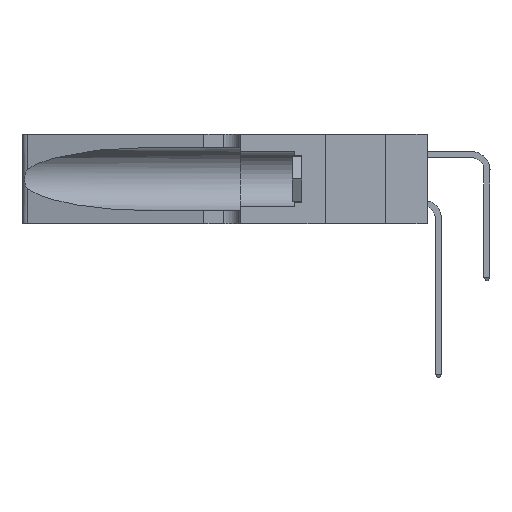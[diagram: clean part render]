
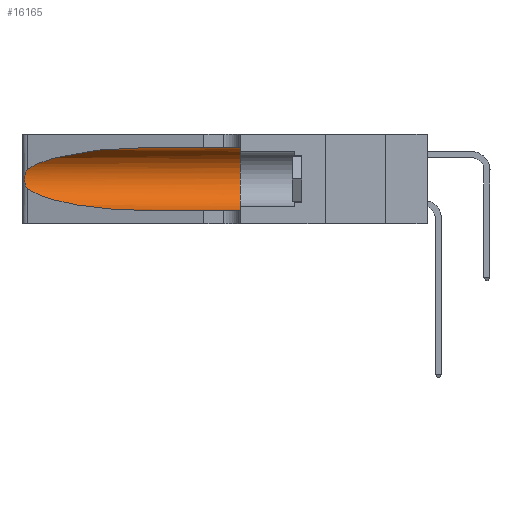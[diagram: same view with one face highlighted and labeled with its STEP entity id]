
A CAD part, left-side view. The second image highlights one B-rep face of the part: STEP entity #16165.
In plain terms, the highlighted cylindrical face has radius 3.308 mm (diameter 6.617 mm), a partial arc.
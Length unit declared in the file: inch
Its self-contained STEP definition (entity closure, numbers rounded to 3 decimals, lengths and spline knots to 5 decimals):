
#218 = VECTOR ( 'NONE', #19047, 39.37008 ) ;
#961 = LINE ( 'NONE', #16708, #218 ) ;
#1011 = B_SPLINE_CURVE_WITH_KNOTS ( 'NONE', 3,
 ( #8698, #10988, #27012, #13292, #29279, #15613, #1794, #17951, #4158, #20252, #6467, #22517, #8791, #24831 ),
 .UNSPECIFIED., .F., .F.,
 ( 4, 2, 2, 2, 2, 2, 4 ),
 ( 0., 0.00027, 0.00053, 0.00107, 0.0016, 0.00187, 0.00214 ),
 .UNSPECIFIED. ) ;
#1794 = CARTESIAN_POINT ( 'NONE',  ( 0.26075, 1.23896, 0.19203 ) ) ;
#2003 = EDGE_LOOP ( 'NONE', ( #27450, #5234, #14921, #28518, #14571, #28187 ) ) ;
#2371 = CARTESIAN_POINT ( 'NONE',  ( 0.2373, 1.15595, 0.08982 ) ) ;
#3690 = FACE_OUTER_BOUND ( 'NONE', #2003, .T. ) ;
#4009 = DIRECTION ( 'NONE',  ( 0., -1., 0. ) ) ;
#4158 = CARTESIAN_POINT ( 'NONE',  ( 0.26017, 1.23833, 0.17102 ) ) ;
#4288 = VECTOR ( 'NONE', #4009, 39.37008 ) ;
#4732 = CARTESIAN_POINT ( 'NONE',  ( 0.25487, 1.22718, 0.14631 ) ) ;
#4951 = AXIS2_PLACEMENT_3D ( 'NONE', #19321, #5542, #21601 ) ;
#5097 = VERTEX_POINT ( 'NONE', #6331 ) ;
#5208 = AXIS2_PLACEMENT_3D ( 'NONE', #8575, #22300, #10869 ) ;
#5234 = ORIENTED_EDGE ( 'NONE', *, *, #7033, .T. ) ;
#5542 = DIRECTION ( 'NONE',  ( 0., 1., 0. ) ) ;
#6032 = CARTESIAN_POINT ( 'NONE',  ( 0.1305, 0.35, 0.31525 ) ) ;
#6320 = VERTEX_POINT ( 'NONE', #28632 ) ;
#6331 = CARTESIAN_POINT ( 'NONE',  ( 0.25487, 1.22718, 0.14631 ) ) ;
#6467 = CARTESIAN_POINT ( 'NONE',  ( 0.25789, 1.23486, 0.15765 ) ) ;
#7033 = EDGE_CURVE ( 'NONE', #21579, #5097, #1011, .T. ) ;
#7039 = CARTESIAN_POINT ( 'NONE',  ( 0.18966, 0.96281, 0.05475 ) ) ;
#7340 =( BOUNDED_CURVE ( )  B_SPLINE_CURVE ( 3, ( #4732, #2371, #7039, #23074 ),
 .UNSPECIFIED., .F., .F. ) 
 B_SPLINE_CURVE_WITH_KNOTS ( ( 4, 4 ),
 ( 3.44316, 4.71239 ),
 .UNSPECIFIED. ) 
 CURVE ( )  GEOMETRIC_REPRESENTATION_ITEM ( )  RATIONAL_B_SPLINE_CURVE ( ( 1., 0.87, 0.87, 1. ) ) 
 REPRESENTATION_ITEM ( '' )  );
#7414 = EDGE_CURVE ( 'NONE', #19714, #10796, #9187, .T. ) ;
#8575 = CARTESIAN_POINT ( 'NONE',  ( 0.1305, 1.61858, 0.185 ) ) ;
#8698 = CARTESIAN_POINT ( 'NONE',  ( 0.25487, 1.22718, 0.22369 ) ) ;
#8791 = CARTESIAN_POINT ( 'NONE',  ( 0.25555, 1.22993, 0.14849 ) ) ;
#8908 = CARTESIAN_POINT ( 'NONE',  ( 0.1305, 0.72297, 0.31525 ) ) ;
#9187 = CIRCLE ( 'NONE', #4951, 0.13025 ) ;
#10379 = LINE ( 'NONE', #13126, #4288 ) ;
#10596 = VERTEX_POINT ( 'NONE', #10965 ) ;
#10796 = VERTEX_POINT ( 'NONE', #13853 ) ;
#10869 = DIRECTION ( 'NONE',  ( 0., 0., -1. ) ) ;
#10965 = CARTESIAN_POINT ( 'NONE',  ( 0.1305, 0.72297, 0.05475 ) ) ;
#10988 = CARTESIAN_POINT ( 'NONE',  ( 0.25555, 1.22994, 0.2215 ) ) ;
#11303 = CARTESIAN_POINT ( 'NONE',  ( 0.25487, 1.22718, 0.22369 ) ) ;
#13126 = CARTESIAN_POINT ( 'NONE',  ( 0.1305, 1.61858, 0.31525 ) ) ;
#13292 = CARTESIAN_POINT ( 'NONE',  ( 0.25787, 1.23484, 0.2124 ) ) ;
#13853 = CARTESIAN_POINT ( 'NONE',  ( 0.1305, 0.35, 0.05475 ) ) ;
#14571 = ORIENTED_EDGE ( 'NONE', *, *, #7414, .F. ) ;
#14838 = CARTESIAN_POINT ( 'NONE',  ( 0.25487, 1.22718, 0.22369 ) ) ;
#14921 = ORIENTED_EDGE ( 'NONE', *, *, #28726, .T. ) ;
#15210 = CYLINDRICAL_SURFACE ( 'NONE', #5208, 0.13025 ) ;
#15613 = CARTESIAN_POINT ( 'NONE',  ( 0.26018, 1.23835, 0.19895 ) ) ;
#16165 = ADVANCED_FACE ( 'NONE', ( #3690 ), #15210, .F. ) ;
#16708 = CARTESIAN_POINT ( 'NONE',  ( 0.1305, 1.61858, 0.05475 ) ) ;
#17951 = CARTESIAN_POINT ( 'NONE',  ( 0.26075, 1.23896, 0.178 ) ) ;
#18410 = EDGE_CURVE ( 'NONE', #6320, #19714, #10379, .T. ) ;
#19047 = DIRECTION ( 'NONE',  ( 0., -1., 0. ) ) ;
#19321 = CARTESIAN_POINT ( 'NONE',  ( 0.1305, 0.35, 0.185 ) ) ;
#19714 = VERTEX_POINT ( 'NONE', #6032 ) ;
#20252 = CARTESIAN_POINT ( 'NONE',  ( 0.25856, 1.23593, 0.16098 ) ) ;
#21579 = VERTEX_POINT ( 'NONE', #14838 ) ;
#21601 = DIRECTION ( 'NONE',  ( 0., 0., 1. ) ) ;
#22300 = DIRECTION ( 'NONE',  ( 0., -1., 0. ) ) ;
#22517 = CARTESIAN_POINT ( 'NONE',  ( 0.25639, 1.23186, 0.15144 ) ) ;
#22736 = CARTESIAN_POINT ( 'NONE',  ( 0.18966, 0.96281, 0.31525 ) ) ;
#23074 = CARTESIAN_POINT ( 'NONE',  ( 0.1305, 0.72297, 0.05475 ) ) ;
#23334 =( BOUNDED_CURVE ( )  B_SPLINE_CURVE ( 3, ( #8908, #22736, #25045, #11303 ),
 .UNSPECIFIED., .F., .F. ) 
 B_SPLINE_CURVE_WITH_KNOTS ( ( 4, 4 ),
 ( 1.5708, 2.84003 ),
 .UNSPECIFIED. ) 
 CURVE ( )  GEOMETRIC_REPRESENTATION_ITEM ( )  RATIONAL_B_SPLINE_CURVE ( ( 1., 0.87, 0.87, 1. ) ) 
 REPRESENTATION_ITEM ( '' )  );
#23930 = EDGE_CURVE ( 'NONE', #6320, #21579, #23334, .T. ) ;
#24520 = EDGE_CURVE ( 'NONE', #10596, #10796, #961, .T. ) ;
#24831 = CARTESIAN_POINT ( 'NONE',  ( 0.25487, 1.22718, 0.14631 ) ) ;
#25045 = CARTESIAN_POINT ( 'NONE',  ( 0.2373, 1.15595, 0.28018 ) ) ;
#27012 = CARTESIAN_POINT ( 'NONE',  ( 0.25639, 1.23184, 0.21858 ) ) ;
#27450 = ORIENTED_EDGE ( 'NONE', *, *, #23930, .T. ) ;
#28187 = ORIENTED_EDGE ( 'NONE', *, *, #18410, .F. ) ;
#28518 = ORIENTED_EDGE ( 'NONE', *, *, #24520, .T. ) ;
#28632 = CARTESIAN_POINT ( 'NONE',  ( 0.1305, 0.72297, 0.31525 ) ) ;
#28726 = EDGE_CURVE ( 'NONE', #5097, #10596, #7340, .T. ) ;
#29279 = CARTESIAN_POINT ( 'NONE',  ( 0.25854, 1.2359, 0.20912 ) ) ;
